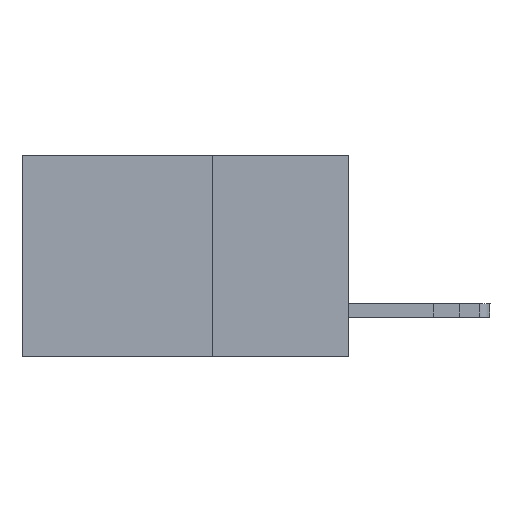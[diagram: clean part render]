
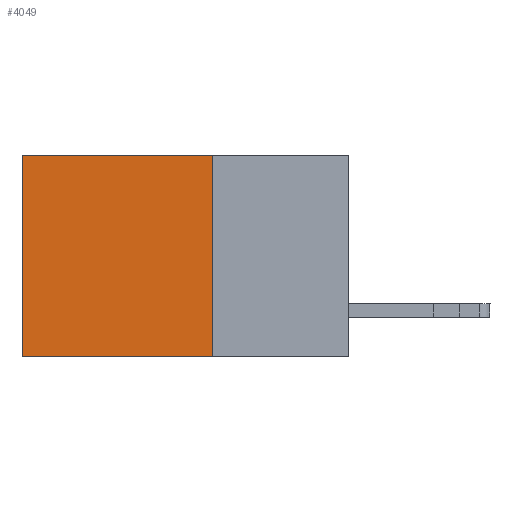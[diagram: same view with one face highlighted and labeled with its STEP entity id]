
A CAD part, left-side view. The second image highlights one B-rep face of the part: STEP entity #4049.
In plain terms, the highlighted planar face has unit normal (-1, 0, 0).
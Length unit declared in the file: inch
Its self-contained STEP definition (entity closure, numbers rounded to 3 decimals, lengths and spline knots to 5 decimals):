
#224 = VERTEX_POINT ( 'NONE', #5719 ) ;
#519 = CARTESIAN_POINT ( 'NONE',  ( 0.2615, 0.6, 0. ) ) ;
#587 = DIRECTION ( 'NONE',  ( 0., 0., -1. ) ) ;
#766 = ORIENTED_EDGE ( 'NONE', *, *, #7043, .F. ) ;
#940 = DIRECTION ( 'NONE',  ( 0., 0., -1. ) ) ;
#1031 = DIRECTION ( 'NONE',  ( 0., 0., -1. ) ) ;
#1944 = LINE ( 'NONE', #4391, #9445 ) ;
#2367 = ORIENTED_EDGE ( 'NONE', *, *, #13834, .T. ) ;
#3495 = ORIENTED_EDGE ( 'NONE', *, *, #14351, .T. ) ;
#3519 = CARTESIAN_POINT ( 'NONE',  ( 0.2615, 0.6, -0.37 ) ) ;
#4049 = ADVANCED_FACE ( 'NONE', ( #11309 ), #11228, .F. ) ;
#4350 = CARTESIAN_POINT ( 'NONE',  ( 0.2615, 0.25, -0.37 ) ) ;
#4391 = CARTESIAN_POINT ( 'NONE',  ( 0.2615, 0.25, -0.37 ) ) ;
#4531 = CARTESIAN_POINT ( 'NONE',  ( 0.2615, 0.25, 0. ) ) ;
#4675 = VERTEX_POINT ( 'NONE', #4531 ) ;
#4744 = CARTESIAN_POINT ( 'NONE',  ( 0.2615, 0.25, -0.37 ) ) ;
#5177 = VECTOR ( 'NONE', #587, 39.37008 ) ;
#5636 = LINE ( 'NONE', #4744, #13847 ) ;
#5719 = CARTESIAN_POINT ( 'NONE',  ( 0.2615, 0.25, -0.37 ) ) ;
#6882 = DIRECTION ( 'NONE',  ( 0., 1., 0. ) ) ;
#7043 = EDGE_CURVE ( 'NONE', #224, #10023, #5636, .T. ) ;
#7306 = VERTEX_POINT ( 'NONE', #519 ) ;
#7325 = DIRECTION ( 'NONE',  ( 0., 1., 0. ) ) ;
#8413 = CARTESIAN_POINT ( 'NONE',  ( 0.2615, 0.25, 0. ) ) ;
#8480 = ORIENTED_EDGE ( 'NONE', *, *, #11229, .F. ) ;
#9445 = VECTOR ( 'NONE', #1031, 39.37008 ) ;
#10023 = VERTEX_POINT ( 'NONE', #3519 ) ;
#10867 = VECTOR ( 'NONE', #7325, 39.37008 ) ;
#10897 = CARTESIAN_POINT ( 'NONE',  ( 0.2615, 0.6, -0.37 ) ) ;
#11228 = PLANE ( 'NONE',  #12266 ) ;
#11229 = EDGE_CURVE ( 'NONE', #4675, #224, #1944, .T. ) ;
#11309 = FACE_OUTER_BOUND ( 'NONE', #12152, .T. ) ;
#11949 = LINE ( 'NONE', #8413, #10867 ) ;
#12152 = EDGE_LOOP ( 'NONE', ( #2367, #766, #8480, #3495 ) ) ;
#12266 = AXIS2_PLACEMENT_3D ( 'NONE', #4350, #12395, #940 ) ;
#12395 = DIRECTION ( 'NONE',  ( 1., 0., 0. ) ) ;
#13834 = EDGE_CURVE ( 'NONE', #7306, #10023, #14273, .T. ) ;
#13847 = VECTOR ( 'NONE', #6882, 39.37008 ) ;
#14273 = LINE ( 'NONE', #10897, #5177 ) ;
#14351 = EDGE_CURVE ( 'NONE', #4675, #7306, #11949, .T. ) ;
